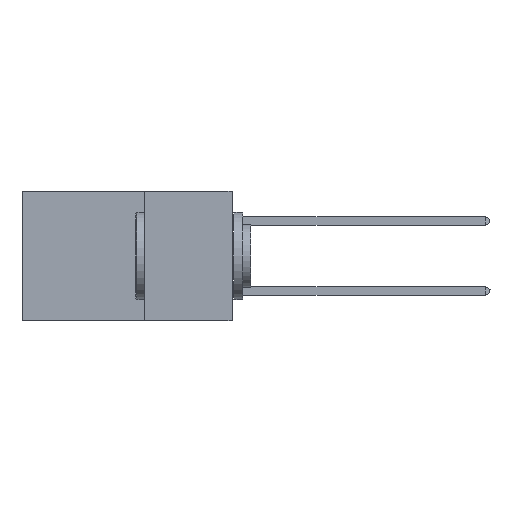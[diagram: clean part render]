
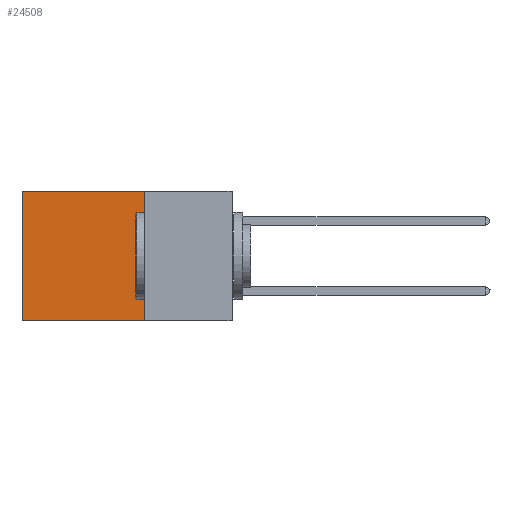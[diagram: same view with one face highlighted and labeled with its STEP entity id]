
A CAD part, left-side view. The second image highlights one B-rep face of the part: STEP entity #24508.
In plain terms, the highlighted planar face has unit normal (-1, 0, 0).
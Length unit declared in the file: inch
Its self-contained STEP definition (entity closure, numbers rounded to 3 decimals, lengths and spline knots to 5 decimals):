
#417 = CARTESIAN_POINT ( 'NONE',  ( 0.2875, 0.25, -0.37 ) ) ;
#1511 = LINE ( 'NONE', #17273, #21879 ) ;
#2330 = DIRECTION ( 'NONE',  ( 0., 1., 0. ) ) ;
#3065 = AXIS2_PLACEMENT_3D ( 'NONE', #26426, #15207, #3683 ) ;
#3177 = CARTESIAN_POINT ( 'NONE',  ( 0.2875, 0.25, 0. ) ) ;
#3683 = DIRECTION ( 'NONE',  ( 0., 0., -1. ) ) ;
#3997 = CARTESIAN_POINT ( 'NONE',  ( 0.2875, 0.6, 0. ) ) ;
#4056 = EDGE_LOOP ( 'NONE', ( #14056, #21964, #18637, #22533 ) ) ;
#4752 = VECTOR ( 'NONE', #2330, 39.37008 ) ;
#6219 = DIRECTION ( 'NONE',  ( 0., 0., -1. ) ) ;
#6739 = LINE ( 'NONE', #3177, #14781 ) ;
#6852 = FACE_OUTER_BOUND ( 'NONE', #4056, .T. ) ;
#6993 = EDGE_CURVE ( 'NONE', #11733, #14402, #1511, .T. ) ;
#8122 = CARTESIAN_POINT ( 'NONE',  ( 0.2875, 0.25, 0. ) ) ;
#11016 = LINE ( 'NONE', #12915, #4752 ) ;
#11733 = VERTEX_POINT ( 'NONE', #3997 ) ;
#12448 = CARTESIAN_POINT ( 'NONE',  ( 0.2875, 0.6, -0.37 ) ) ;
#12915 = CARTESIAN_POINT ( 'NONE',  ( 0.2875, 0.25, -0.37 ) ) ;
#14056 = ORIENTED_EDGE ( 'NONE', *, *, #6993, .T. ) ;
#14402 = VERTEX_POINT ( 'NONE', #12448 ) ;
#14781 = VECTOR ( 'NONE', #27914, 39.37008 ) ;
#14866 = DIRECTION ( 'NONE',  ( 0., 0., -1. ) ) ;
#15188 = EDGE_CURVE ( 'NONE', #21220, #24082, #25934, .T. ) ;
#15207 = DIRECTION ( 'NONE',  ( 1., 0., 0. ) ) ;
#16088 = VECTOR ( 'NONE', #14866, 39.37008 ) ;
#17273 = CARTESIAN_POINT ( 'NONE',  ( 0.2875, 0.6, 0. ) ) ;
#18103 = EDGE_CURVE ( 'NONE', #24082, #14402, #11016, .T. ) ;
#18637 = ORIENTED_EDGE ( 'NONE', *, *, #15188, .F. ) ;
#21220 = VERTEX_POINT ( 'NONE', #25883 ) ;
#21800 = EDGE_CURVE ( 'NONE', #21220, #11733, #6739, .T. ) ;
#21879 = VECTOR ( 'NONE', #6219, 39.37008 ) ;
#21964 = ORIENTED_EDGE ( 'NONE', *, *, #18103, .F. ) ;
#22533 = ORIENTED_EDGE ( 'NONE', *, *, #21800, .T. ) ;
#24082 = VERTEX_POINT ( 'NONE', #417 ) ;
#24508 = ADVANCED_FACE ( 'NONE', ( #6852 ), #28588, .F. ) ;
#25883 = CARTESIAN_POINT ( 'NONE',  ( 0.2875, 0.25, 0. ) ) ;
#25934 = LINE ( 'NONE', #8122, #16088 ) ;
#26426 = CARTESIAN_POINT ( 'NONE',  ( 0.2875, 0.25, 0. ) ) ;
#27914 = DIRECTION ( 'NONE',  ( 0., 1., 0. ) ) ;
#28588 = PLANE ( 'NONE',  #3065 ) ;
